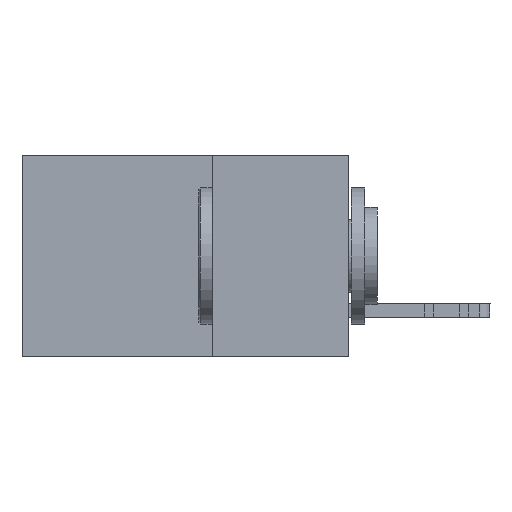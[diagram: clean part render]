
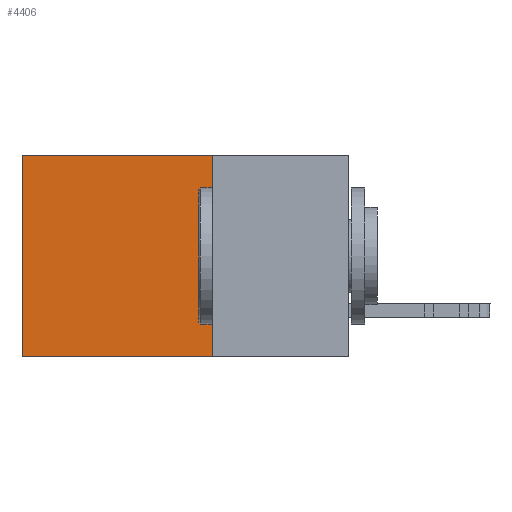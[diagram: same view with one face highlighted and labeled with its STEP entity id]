
A CAD part, left-side view. The second image highlights one B-rep face of the part: STEP entity #4406.
In plain terms, the highlighted planar face has unit normal (-1, 0, 0).
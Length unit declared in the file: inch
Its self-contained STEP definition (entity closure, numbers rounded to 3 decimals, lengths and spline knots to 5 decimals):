
#992 = VERTEX_POINT ( 'NONE', #12958 ) ;
#3118 = EDGE_CURVE ( 'NONE', #20837, #7718, #16940, .T. ) ;
#3268 = FACE_OUTER_BOUND ( 'NONE', #25607, .T. ) ;
#4079 = VERTEX_POINT ( 'NONE', #20803 ) ;
#4406 = ADVANCED_FACE ( 'NONE', ( #3268 ), #11586, .F. ) ;
#4589 = ORIENTED_EDGE ( 'NONE', *, *, #3118, .F. ) ;
#6158 = DIRECTION ( 'NONE',  ( 0., 1., 0. ) ) ;
#6407 = ORIENTED_EDGE ( 'NONE', *, *, #11977, .T. ) ;
#6409 = VECTOR ( 'NONE', #25661, 39.37008 ) ;
#7316 = CARTESIAN_POINT ( 'NONE',  ( 0.2615, 0.25, -0.37 ) ) ;
#7718 = VERTEX_POINT ( 'NONE', #23021 ) ;
#8095 = CARTESIAN_POINT ( 'NONE',  ( 0.2615, 0.25, 0. ) ) ;
#9067 = CARTESIAN_POINT ( 'NONE',  ( 0.2615, 0.6, -0.37 ) ) ;
#9317 = DIRECTION ( 'NONE',  ( 0., 1., 0. ) ) ;
#10512 = VECTOR ( 'NONE', #9317, 39.37008 ) ;
#10556 = DIRECTION ( 'NONE',  ( 0., 0., -1. ) ) ;
#10826 = DIRECTION ( 'NONE',  ( 1., 0., 0. ) ) ;
#10852 = CARTESIAN_POINT ( 'NONE',  ( 0.2615, 0.25, -0.37 ) ) ;
#11586 = PLANE ( 'NONE',  #15534 ) ;
#11618 = EDGE_CURVE ( 'NONE', #20837, #992, #23906, .T. ) ;
#11977 = EDGE_CURVE ( 'NONE', #992, #4079, #21121, .T. ) ;
#12717 = VECTOR ( 'NONE', #6158, 39.37008 ) ;
#12958 = CARTESIAN_POINT ( 'NONE',  ( 0.2615, 0.6, 0. ) ) ;
#13019 = ORIENTED_EDGE ( 'NONE', *, *, #15234, .F. ) ;
#14835 = ORIENTED_EDGE ( 'NONE', *, *, #11618, .T. ) ;
#15234 = EDGE_CURVE ( 'NONE', #7718, #4079, #25682, .T. ) ;
#15534 = AXIS2_PLACEMENT_3D ( 'NONE', #10852, #10826, #10556 ) ;
#16001 = CARTESIAN_POINT ( 'NONE',  ( 0.2615, 0.25, 0. ) ) ;
#16940 = LINE ( 'NONE', #25578, #6409 ) ;
#18982 = DIRECTION ( 'NONE',  ( 0., 0., -1. ) ) ;
#20803 = CARTESIAN_POINT ( 'NONE',  ( 0.2615, 0.6, -0.37 ) ) ;
#20837 = VERTEX_POINT ( 'NONE', #8095 ) ;
#21121 = LINE ( 'NONE', #9067, #25696 ) ;
#23021 = CARTESIAN_POINT ( 'NONE',  ( 0.2615, 0.25, -0.37 ) ) ;
#23906 = LINE ( 'NONE', #16001, #12717 ) ;
#25578 = CARTESIAN_POINT ( 'NONE',  ( 0.2615, 0.25, -0.37 ) ) ;
#25607 = EDGE_LOOP ( 'NONE', ( #6407, #13019, #4589, #14835 ) ) ;
#25661 = DIRECTION ( 'NONE',  ( 0., 0., -1. ) ) ;
#25682 = LINE ( 'NONE', #7316, #10512 ) ;
#25696 = VECTOR ( 'NONE', #18982, 39.37008 ) ;
